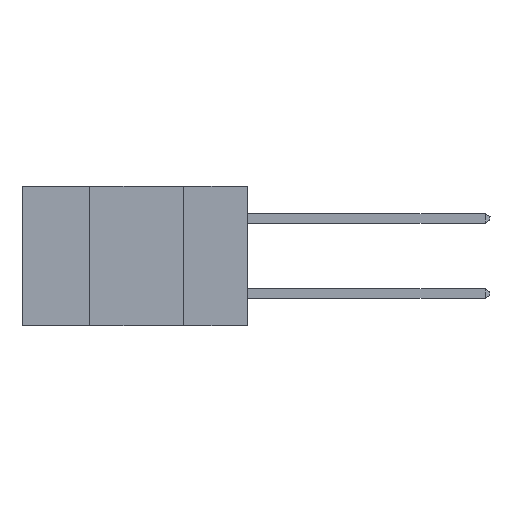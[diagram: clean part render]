
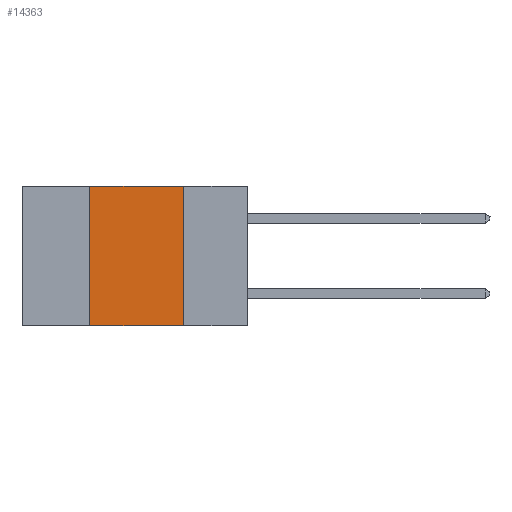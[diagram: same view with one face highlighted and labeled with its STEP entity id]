
A CAD part, left-side view. The second image highlights one B-rep face of the part: STEP entity #14363.
In plain terms, the highlighted planar face has unit normal (-1, 0, 0).
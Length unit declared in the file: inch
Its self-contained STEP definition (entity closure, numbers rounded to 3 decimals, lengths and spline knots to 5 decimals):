
#162 = CARTESIAN_POINT ( 'NONE',  ( 0., 0.17, 0. ) ) ;
#253 = ORIENTED_EDGE ( 'NONE', *, *, #12670, .T. ) ;
#1035 = EDGE_CURVE ( 'NONE', #18220, #23804, #10324, .T. ) ;
#2544 = ORIENTED_EDGE ( 'NONE', *, *, #12201, .F. ) ;
#4266 = FACE_OUTER_BOUND ( 'NONE', #21984, .T. ) ;
#6530 = VECTOR ( 'NONE', #19520, 39.37008 ) ;
#6969 = VECTOR ( 'NONE', #9160, 39.37008 ) ;
#7751 = CARTESIAN_POINT ( 'NONE',  ( 0., 0.17, -0.37 ) ) ;
#9160 = DIRECTION ( 'NONE',  ( 0., 0., -1. ) ) ;
#9825 = CARTESIAN_POINT ( 'NONE',  ( 0., 0.42, 0. ) ) ;
#10145 = CARTESIAN_POINT ( 'NONE',  ( 0., 0.6, 0. ) ) ;
#10324 = LINE ( 'NONE', #10145, #6530 ) ;
#11352 = DIRECTION ( 'NONE',  ( 0., -1., 0. ) ) ;
#12201 = EDGE_CURVE ( 'NONE', #23804, #12817, #17623, .T. ) ;
#12549 = VECTOR ( 'NONE', #29198, 39.37008 ) ;
#12650 = LINE ( 'NONE', #16108, #25560 ) ;
#12670 = EDGE_CURVE ( 'NONE', #25279, #12817, #12650, .T. ) ;
#12817 = VERTEX_POINT ( 'NONE', #7751 ) ;
#14363 = ADVANCED_FACE ( 'NONE', ( #4266 ), #25437, .F. ) ;
#15447 = DIRECTION ( 'NONE',  ( 1., 0., 0. ) ) ;
#15583 = AXIS2_PLACEMENT_3D ( 'NONE', #23118, #15447, #27642 ) ;
#16108 = CARTESIAN_POINT ( 'NONE',  ( 0., 0.6, -0.37 ) ) ;
#16884 = CARTESIAN_POINT ( 'NONE',  ( 0., 0.17, 0. ) ) ;
#17623 = LINE ( 'NONE', #16884, #6969 ) ;
#18220 = VERTEX_POINT ( 'NONE', #30821 ) ;
#19520 = DIRECTION ( 'NONE',  ( 0., -1., 0. ) ) ;
#21984 = EDGE_LOOP ( 'NONE', ( #2544, #28405, #22998, #253 ) ) ;
#22902 = CARTESIAN_POINT ( 'NONE',  ( 0., 0.42, -0.37 ) ) ;
#22998 = ORIENTED_EDGE ( 'NONE', *, *, #26531, .F. ) ;
#23118 = CARTESIAN_POINT ( 'NONE',  ( 0., 0.6, 0. ) ) ;
#23187 = LINE ( 'NONE', #9825, #12549 ) ;
#23804 = VERTEX_POINT ( 'NONE', #162 ) ;
#25279 = VERTEX_POINT ( 'NONE', #22902 ) ;
#25437 = PLANE ( 'NONE',  #15583 ) ;
#25560 = VECTOR ( 'NONE', #11352, 39.37008 ) ;
#26531 = EDGE_CURVE ( 'NONE', #25279, #18220, #23187, .T. ) ;
#27642 = DIRECTION ( 'NONE',  ( 0., 0., -1. ) ) ;
#28405 = ORIENTED_EDGE ( 'NONE', *, *, #1035, .F. ) ;
#29198 = DIRECTION ( 'NONE',  ( 0., 0., 1. ) ) ;
#30821 = CARTESIAN_POINT ( 'NONE',  ( 0., 0.42, 0. ) ) ;
